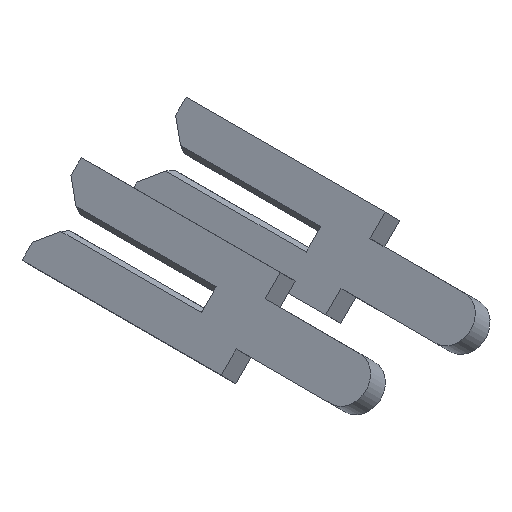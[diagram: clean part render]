
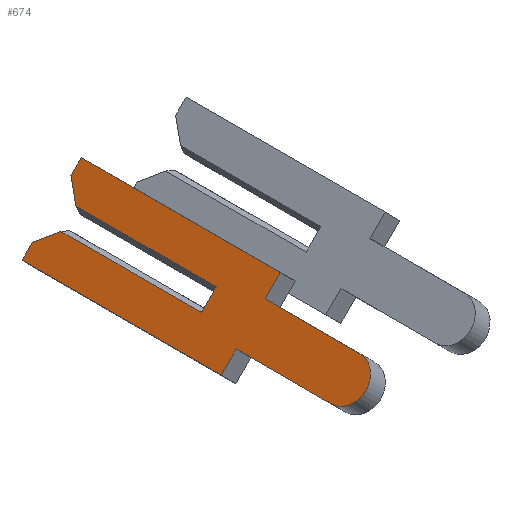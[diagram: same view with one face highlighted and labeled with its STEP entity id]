
A CAD part, isometric view. The second image highlights one B-rep face of the part: STEP entity #674.
In plain terms, the highlighted face is planar.
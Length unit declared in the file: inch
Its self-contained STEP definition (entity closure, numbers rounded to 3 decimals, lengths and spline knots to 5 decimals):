
#14 = VECTOR ( 'NONE', #557, 39.37008 ) ;
#19 = CARTESIAN_POINT ( 'NONE',  ( -0.01, -0.1305, 0. ) ) ;
#29 = CARTESIAN_POINT ( 'NONE',  ( -0.01, -0.1305, 0.0195 ) ) ;
#53 = CARTESIAN_POINT ( 'NONE',  ( -0.01, 0.1305, 0.0065 ) ) ;
#55 = CARTESIAN_POINT ( 'NONE',  ( -0.01, 0.1305, -0.0065 ) ) ;
#57 = CARTESIAN_POINT ( 'NONE',  ( -0.01, -0.04, 0.04 ) ) ;
#60 = VECTOR ( 'NONE', #737, 39.37008 ) ;
#61 = ORIENTED_EDGE ( 'NONE', *, *, #589, .F. ) ;
#63 = LINE ( 'NONE', #317, #543 ) ;
#71 = CARTESIAN_POINT ( 'NONE',  ( -0.01, -0.04, 0.0195 ) ) ;
#76 = ORIENTED_EDGE ( 'NONE', *, *, #406, .F. ) ;
#106 = LINE ( 'NONE', #55, #712 ) ;
#107 = LINE ( 'NONE', #53, #622 ) ;
#120 = VERTEX_POINT ( 'NONE', #29 ) ;
#122 = VERTEX_POINT ( 'NONE', #428 ) ;
#129 = CARTESIAN_POINT ( 'NONE',  ( -0.01, -0.1305, -0.0195 ) ) ;
#139 = EDGE_CURVE ( 'NONE', #414, #199, #210, .T. ) ;
#142 = EDGE_CURVE ( 'NONE', #626, #122, #179, .T. ) ;
#173 = CARTESIAN_POINT ( 'NONE',  ( -0.01, 0.15, -0.04 ) ) ;
#179 = LINE ( 'NONE', #681, #14 ) ;
#180 = LINE ( 'NONE', #320, #503 ) ;
#181 = VECTOR ( 'NONE', #860, 39.37008 ) ;
#197 = DIRECTION ( 'NONE',  ( 0., 0., -1. ) ) ;
#199 = VERTEX_POINT ( 'NONE', #173 ) ;
#206 = ORIENTED_EDGE ( 'NONE', *, *, #569, .F. ) ;
#210 = LINE ( 'NONE', #684, #537 ) ;
#220 = EDGE_CURVE ( 'NONE', #400, #770, #403, .T. ) ;
#242 = EDGE_CURVE ( 'NONE', #462, #558, #63, .T. ) ;
#251 = CARTESIAN_POINT ( 'NONE',  ( -0.01, 0.134, 0.01 ) ) ;
#255 = CARTESIAN_POINT ( 'NONE',  ( -0.01, 0.15, 0.04 ) ) ;
#276 = CARTESIAN_POINT ( 'NONE',  ( -0.01, -0.1305, 0. ) ) ;
#282 = CARTESIAN_POINT ( 'NONE',  ( -0.01, -0.04, -0.0195 ) ) ;
#288 = VECTOR ( 'NONE', #769, 39.37008 ) ;
#304 = ORIENTED_EDGE ( 'NONE', *, *, #242, .T. ) ;
#317 = CARTESIAN_POINT ( 'NONE',  ( -0.01, 0.15, 0.01 ) ) ;
#320 = CARTESIAN_POINT ( 'NONE',  ( -0.01, -0.04, 0.0195 ) ) ;
#340 = LINE ( 'NONE', #57, #846 ) ;
#344 = EDGE_CURVE ( 'NONE', #535, #120, #180, .T. ) ;
#353 = CARTESIAN_POINT ( 'NONE',  ( -0.01, 0.134, -0.01 ) ) ;
#354 = CARTESIAN_POINT ( 'NONE',  ( -0.01, 0.15, 0.026 ) ) ;
#360 = EDGE_CURVE ( 'NONE', #666, #626, #106, .T. ) ;
#370 = ORIENTED_EDGE ( 'NONE', *, *, #385, .F. ) ;
#380 = EDGE_CURVE ( 'NONE', #458, #535, #340, .T. ) ;
#385 = EDGE_CURVE ( 'NONE', #636, #442, #440, .T. ) ;
#400 = VERTEX_POINT ( 'NONE', #129 ) ;
#403 = LINE ( 'NONE', #705, #288 ) ;
#406 = EDGE_CURVE ( 'NONE', #462, #636, #107, .T. ) ;
#414 = VERTEX_POINT ( 'NONE', #849 ) ;
#416 = EDGE_CURVE ( 'NONE', #442, #458, #478, .T. ) ;
#422 = EDGE_CURVE ( 'NONE', #770, #414, #835, .T. ) ;
#423 = CARTESIAN_POINT ( 'NONE',  ( -0.01, 0.15, -0.026 ) ) ;
#424 = DIRECTION ( 'NONE',  ( 1., 0., 0. ) ) ;
#428 = CARTESIAN_POINT ( 'NONE',  ( -0.01, 0., -0.01 ) ) ;
#434 = ORIENTED_EDGE ( 'NONE', *, *, #416, .F. ) ;
#440 = LINE ( 'NONE', #650, #181 ) ;
#442 = VERTEX_POINT ( 'NONE', #255 ) ;
#447 = VECTOR ( 'NONE', #689, 39.37008 ) ;
#448 = DIRECTION ( 'NONE',  ( 0., -0.707, 0.707 ) ) ;
#451 = ORIENTED_EDGE ( 'NONE', *, *, #220, .F. ) ;
#458 = VERTEX_POINT ( 'NONE', #851 ) ;
#462 = VERTEX_POINT ( 'NONE', #251 ) ;
#471 = ORIENTED_EDGE ( 'NONE', *, *, #344, .F. ) ;
#478 = LINE ( 'NONE', #507, #447 ) ;
#503 = VECTOR ( 'NONE', #788, 39.37008 ) ;
#507 = CARTESIAN_POINT ( 'NONE',  ( -0.01, 0.15, 0.04 ) ) ;
#518 = CARTESIAN_POINT ( 'NONE',  ( -0.01, -0.04, -0.04 ) ) ;
#522 = AXIS2_PLACEMENT_3D ( 'NONE', #19, #424, #613 ) ;
#524 = DIRECTION ( 'NONE',  ( 1., 0., 0. ) ) ;
#527 = CARTESIAN_POINT ( 'NONE',  ( -0.01, 0., 0.01 ) ) ;
#535 = VERTEX_POINT ( 'NONE', #71 ) ;
#537 = VECTOR ( 'NONE', #614, 39.37008 ) ;
#539 = CARTESIAN_POINT ( 'NONE',  ( -0.01, 0.15, -0.026 ) ) ;
#543 = VECTOR ( 'NONE', #634, 39.37008 ) ;
#551 = LINE ( 'NONE', #539, #60 ) ;
#557 = DIRECTION ( 'NONE',  ( 0., -1., 0. ) ) ;
#558 = VERTEX_POINT ( 'NONE', #527 ) ;
#566 = VECTOR ( 'NONE', #646, 39.37008 ) ;
#569 = EDGE_CURVE ( 'NONE', #120, #400, #694, .T. ) ;
#588 = CARTESIAN_POINT ( 'NONE',  ( -0.01, 0., 0.0065 ) ) ;
#589 = EDGE_CURVE ( 'NONE', #122, #558, #660, .T. ) ;
#613 = DIRECTION ( 'NONE',  ( 0., 0., -1. ) ) ;
#614 = DIRECTION ( 'NONE',  ( 0., 1., 0. ) ) ;
#622 = VECTOR ( 'NONE', #857, 39.37008 ) ;
#626 = VERTEX_POINT ( 'NONE', #353 ) ;
#634 = DIRECTION ( 'NONE',  ( 0., -1., 0. ) ) ;
#636 = VERTEX_POINT ( 'NONE', #354 ) ;
#646 = DIRECTION ( 'NONE',  ( 0., 0., -1. ) ) ;
#650 = CARTESIAN_POINT ( 'NONE',  ( -0.01, 0.15, 0.026 ) ) ;
#660 = LINE ( 'NONE', #588, #817 ) ;
#666 = VERTEX_POINT ( 'NONE', #423 ) ;
#674 = ADVANCED_FACE ( 'NONE', ( #734 ), #810, .F. ) ;
#675 = EDGE_CURVE ( 'NONE', #199, #666, #551, .T. ) ;
#681 = CARTESIAN_POINT ( 'NONE',  ( -0.01, -0.1305, -0.01 ) ) ;
#684 = CARTESIAN_POINT ( 'NONE',  ( -0.01, 0.15, -0.04 ) ) ;
#689 = DIRECTION ( 'NONE',  ( 0., -1., 0. ) ) ;
#694 = CIRCLE ( 'NONE', #848, 0.0195 ) ;
#705 = CARTESIAN_POINT ( 'NONE',  ( -0.01, -0.04, -0.0195 ) ) ;
#712 = VECTOR ( 'NONE', #448, 39.37008 ) ;
#728 = DIRECTION ( 'NONE',  ( 0., 0., 1. ) ) ;
#732 = ORIENTED_EDGE ( 'NONE', *, *, #142, .F. ) ;
#734 = FACE_OUTER_BOUND ( 'NONE', #784, .T. ) ;
#737 = DIRECTION ( 'NONE',  ( 0., 0., 1. ) ) ;
#739 = ORIENTED_EDGE ( 'NONE', *, *, #422, .F. ) ;
#761 = ORIENTED_EDGE ( 'NONE', *, *, #675, .F. ) ;
#769 = DIRECTION ( 'NONE',  ( 0., 1., 0. ) ) ;
#770 = VERTEX_POINT ( 'NONE', #282 ) ;
#784 = EDGE_LOOP ( 'NONE', ( #304, #61, #732, #841, #761, #853, #739, #451, #206, #471, #823, #434, #370, #76 ) ) ;
#788 = DIRECTION ( 'NONE',  ( 0., -1., 0. ) ) ;
#796 = DIRECTION ( 'NONE',  ( 0., 0., -1. ) ) ;
#810 = PLANE ( 'NONE',  #522 ) ;
#817 = VECTOR ( 'NONE', #728, 39.37008 ) ;
#823 = ORIENTED_EDGE ( 'NONE', *, *, #380, .F. ) ;
#835 = LINE ( 'NONE', #518, #566 ) ;
#841 = ORIENTED_EDGE ( 'NONE', *, *, #360, .F. ) ;
#846 = VECTOR ( 'NONE', #197, 39.37008 ) ;
#848 = AXIS2_PLACEMENT_3D ( 'NONE', #276, #524, #796 ) ;
#849 = CARTESIAN_POINT ( 'NONE',  ( -0.01, -0.04, -0.04 ) ) ;
#851 = CARTESIAN_POINT ( 'NONE',  ( -0.01, -0.04, 0.04 ) ) ;
#853 = ORIENTED_EDGE ( 'NONE', *, *, #139, .F. ) ;
#857 = DIRECTION ( 'NONE',  ( 0., 0.707, 0.707 ) ) ;
#860 = DIRECTION ( 'NONE',  ( 0., 0., 1. ) ) ;
